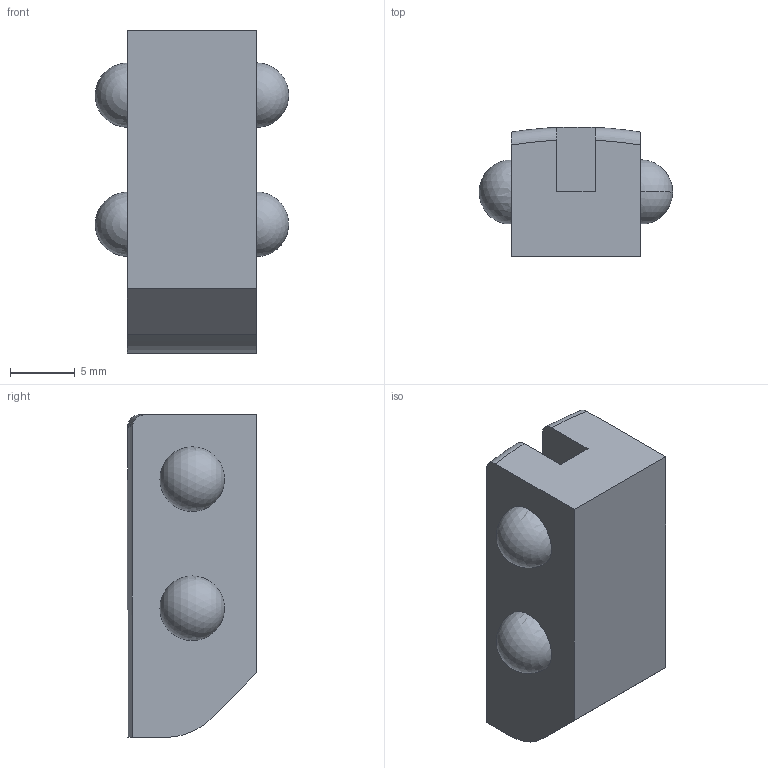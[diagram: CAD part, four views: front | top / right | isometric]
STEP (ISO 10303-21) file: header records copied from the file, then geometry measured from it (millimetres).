
FILE_DESCRIPTION (( 'STEP AP214' ), '1' );
FILE_NAME ('Top_Cover.STEP', '2013-11-21T02:42:38', ( '' ), ( '' ), 'SwSTEP 2.0', 'SolidWorks 2013', '' );
FILE_SCHEMA (( 'AUTOMOTIVE_DESIGN' ));
Length unit declared in the file: millimetre
Products named in the file (1): Top_Cover
Bounding box: 14.98 x 10.03 x 25 mm (x, y, z)
Volume: 2398.9 mm3; surface area: 1247.9 mm2
Topology: 1 solids, 1 shells, 20 faces, 62 edges, 40 vertices
Faces by surface type: plane 10, sphere 6, torus 2, cylinder 2
Entity records: 640 total; most frequent: CARTESIAN_POINT 133, DIRECTION 102, ORIENTED_EDGE 92, EDGE_CURVE 46, AXIS2_PLACEMENT_3D 39, VERTEX_POINT 32, VECTOR 24, LINE 24
